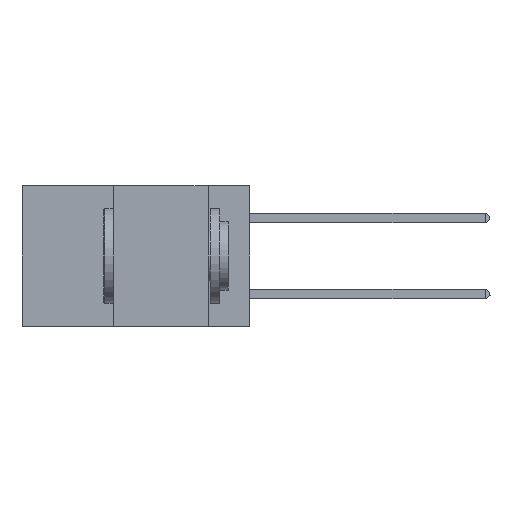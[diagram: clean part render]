
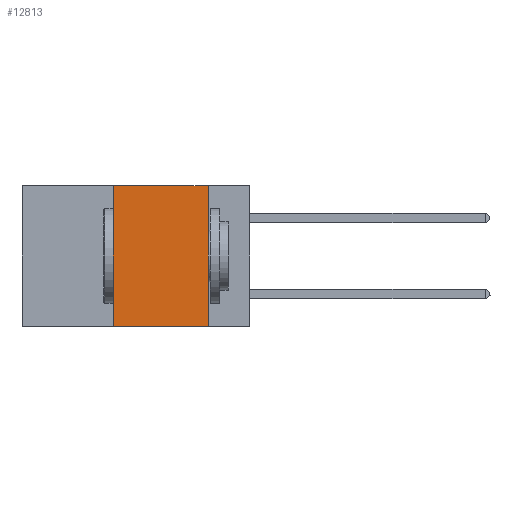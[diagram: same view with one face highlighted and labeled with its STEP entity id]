
A CAD part, left-side view. The second image highlights one B-rep face of the part: STEP entity #12813.
In plain terms, the highlighted planar face has unit normal (-1, 0, 0).
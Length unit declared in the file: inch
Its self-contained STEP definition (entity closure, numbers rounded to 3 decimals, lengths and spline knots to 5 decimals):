
#1002 = FACE_OUTER_BOUND ( 'NONE', #12924, .T. ) ;
#2160 = VECTOR ( 'NONE', #14866, 39.37008 ) ;
#2458 = EDGE_CURVE ( 'NONE', #3597, #16422, #6546, .T. ) ;
#3597 = VERTEX_POINT ( 'NONE', #11503 ) ;
#3932 = CARTESIAN_POINT ( 'NONE',  ( 0., 0.36, 0. ) ) ;
#4191 = CARTESIAN_POINT ( 'NONE',  ( 0., 0.6, 0. ) ) ;
#4572 = CARTESIAN_POINT ( 'NONE',  ( 0., 0.36, -0.37 ) ) ;
#6294 = EDGE_CURVE ( 'NONE', #15377, #12564, #14347, .T. ) ;
#6546 = LINE ( 'NONE', #16537, #11224 ) ;
#6592 = EDGE_CURVE ( 'NONE', #15377, #16422, #7623, .T. ) ;
#7623 = LINE ( 'NONE', #13157, #13717 ) ;
#8331 = CARTESIAN_POINT ( 'NONE',  ( 0., 0.36, 0. ) ) ;
#9336 = VECTOR ( 'NONE', #14719, 39.37008 ) ;
#9546 = AXIS2_PLACEMENT_3D ( 'NONE', #4191, #14416, #10509 ) ;
#10035 = CARTESIAN_POINT ( 'NONE',  ( 0., 0.11, -0.37 ) ) ;
#10379 = ORIENTED_EDGE ( 'NONE', *, *, #13094, .F. ) ;
#10509 = DIRECTION ( 'NONE',  ( 0., 0., -1. ) ) ;
#10554 = DIRECTION ( 'NONE',  ( 0., -1., 0. ) ) ;
#10684 = PLANE ( 'NONE',  #9546 ) ;
#11001 = CARTESIAN_POINT ( 'NONE',  ( 0., 0.6, 0. ) ) ;
#11224 = VECTOR ( 'NONE', #12887, 39.37008 ) ;
#11503 = CARTESIAN_POINT ( 'NONE',  ( 0., 0.11, 0. ) ) ;
#11821 = ORIENTED_EDGE ( 'NONE', *, *, #6592, .T. ) ;
#12564 = VERTEX_POINT ( 'NONE', #3932 ) ;
#12624 = ORIENTED_EDGE ( 'NONE', *, *, #6294, .F. ) ;
#12813 = ADVANCED_FACE ( 'NONE', ( #1002 ), #10684, .F. ) ;
#12887 = DIRECTION ( 'NONE',  ( 0., 0., -1. ) ) ;
#12924 = EDGE_LOOP ( 'NONE', ( #15798, #10379, #12624, #11821 ) ) ;
#13094 = EDGE_CURVE ( 'NONE', #12564, #3597, #13203, .T. ) ;
#13157 = CARTESIAN_POINT ( 'NONE',  ( 0., 0.6, -0.37 ) ) ;
#13203 = LINE ( 'NONE', #11001, #9336 ) ;
#13717 = VECTOR ( 'NONE', #10554, 39.37008 ) ;
#14347 = LINE ( 'NONE', #8331, #2160 ) ;
#14416 = DIRECTION ( 'NONE',  ( 1., 0., 0. ) ) ;
#14719 = DIRECTION ( 'NONE',  ( 0., -1., 0. ) ) ;
#14866 = DIRECTION ( 'NONE',  ( 0., 0., 1. ) ) ;
#15377 = VERTEX_POINT ( 'NONE', #4572 ) ;
#15798 = ORIENTED_EDGE ( 'NONE', *, *, #2458, .F. ) ;
#16422 = VERTEX_POINT ( 'NONE', #10035 ) ;
#16537 = CARTESIAN_POINT ( 'NONE',  ( 0., 0.11, 0. ) ) ;
